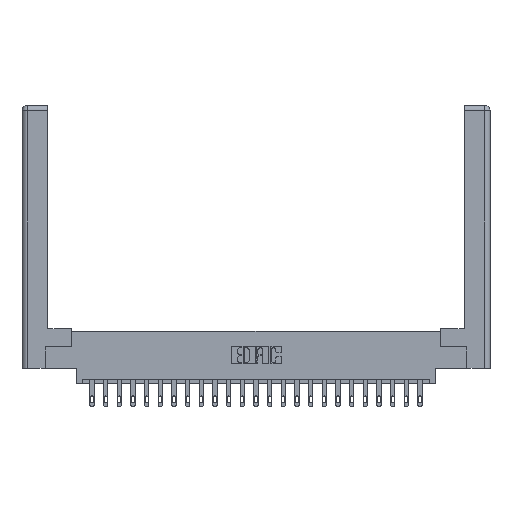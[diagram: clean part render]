
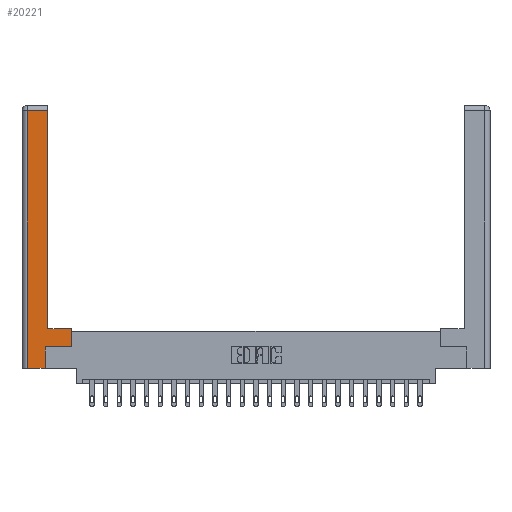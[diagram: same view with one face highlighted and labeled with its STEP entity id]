
A CAD part, top view. The second image highlights one B-rep face of the part: STEP entity #20221.
In plain terms, the highlighted planar face has unit normal (0, 0, 1).
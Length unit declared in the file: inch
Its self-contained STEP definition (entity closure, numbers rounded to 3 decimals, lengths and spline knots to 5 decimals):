
#418 = VECTOR ( 'NONE', #13907, 39.37008 ) ;
#998 = DIRECTION ( 'NONE',  ( 0., 0., -1. ) ) ;
#1299 = VECTOR ( 'NONE', #5932, 39.37008 ) ;
#1701 = LINE ( 'NONE', #20860, #18689 ) ;
#2306 = DIRECTION ( 'NONE',  ( 1., 0., 0. ) ) ;
#2366 = ORIENTED_EDGE ( 'NONE', *, *, #10690, .T. ) ;
#2379 = CARTESIAN_POINT ( 'NONE',  ( 0.565, 0.245, 0. ) ) ;
#2424 = VERTEX_POINT ( 'NONE', #11242 ) ;
#2531 = VERTEX_POINT ( 'NONE', #2379 ) ;
#2555 = EDGE_CURVE ( 'NONE', #7389, #2424, #16528, .T. ) ;
#3849 = DIRECTION ( 'NONE',  ( 0., 1., 0. ) ) ;
#3853 = FACE_OUTER_BOUND ( 'NONE', #3974, .T. ) ;
#3923 = CARTESIAN_POINT ( 'NONE',  ( 0.265, 0.245, 0. ) ) ;
#3974 = EDGE_LOOP ( 'NONE', ( #2366, #7760, #23906, #14959, #4752, #15238, #15988, #21761 ) ) ;
#4014 = CARTESIAN_POINT ( 'NONE',  ( 0.0615, 0., 0. ) ) ;
#4451 = CARTESIAN_POINT ( 'NONE',  ( 0.0615, 2.94, 0. ) ) ;
#4752 = ORIENTED_EDGE ( 'NONE', *, *, #21099, .T. ) ;
#5084 = EDGE_CURVE ( 'NONE', #19038, #7389, #6568, .T. ) ;
#5932 = DIRECTION ( 'NONE',  ( 0., 1., 0. ) ) ;
#6568 = LINE ( 'NONE', #4451, #418 ) ;
#7389 = VERTEX_POINT ( 'NONE', #16466 ) ;
#7545 = DIRECTION ( 'NONE',  ( 0., 1., 0. ) ) ;
#7642 = CARTESIAN_POINT ( 'NONE',  ( 0.265, 0., 0. ) ) ;
#7760 = ORIENTED_EDGE ( 'NONE', *, *, #5084, .T. ) ;
#8191 = VERTEX_POINT ( 'NONE', #22453 ) ;
#8256 = EDGE_CURVE ( 'NONE', #23671, #8191, #20503, .T. ) ;
#8374 = PLANE ( 'NONE',  #10267 ) ;
#8852 = CARTESIAN_POINT ( 'NONE',  ( 0.265, 0.245, 0. ) ) ;
#9056 = LINE ( 'NONE', #3923, #13434 ) ;
#9840 = DIRECTION ( 'NONE',  ( -1., 0., 0. ) ) ;
#10085 = VECTOR ( 'NONE', #2306, 39.37008 ) ;
#10267 = AXIS2_PLACEMENT_3D ( 'NONE', #16216, #998, #14243 ) ;
#10690 = EDGE_CURVE ( 'NONE', #8191, #19038, #10992, .T. ) ;
#10992 = LINE ( 'NONE', #15059, #1299 ) ;
#11045 = CARTESIAN_POINT ( 'NONE',  ( 0.295, 2.94, 0. ) ) ;
#11242 = CARTESIAN_POINT ( 'NONE',  ( 0.0615, 0., 0. ) ) ;
#13253 = CARTESIAN_POINT ( 'NONE',  ( 0.565, 0.45, 0. ) ) ;
#13434 = VECTOR ( 'NONE', #3849, 39.37008 ) ;
#13907 = DIRECTION ( 'NONE',  ( -1., 0., 0. ) ) ;
#14243 = DIRECTION ( 'NONE',  ( -1., 0., 0. ) ) ;
#14959 = ORIENTED_EDGE ( 'NONE', *, *, #18360, .T. ) ;
#15059 = CARTESIAN_POINT ( 'NONE',  ( 0.295, 3., 0. ) ) ;
#15110 = DIRECTION ( 'NONE',  ( 1., 0., 0. ) ) ;
#15238 = ORIENTED_EDGE ( 'NONE', *, *, #21223, .T. ) ;
#15934 = VERTEX_POINT ( 'NONE', #16147 ) ;
#15988 = ORIENTED_EDGE ( 'NONE', *, *, #16335, .T. ) ;
#16147 = CARTESIAN_POINT ( 'NONE',  ( 0.265, 0., 0. ) ) ;
#16216 = CARTESIAN_POINT ( 'NONE',  ( 0., 0., 0. ) ) ;
#16335 = EDGE_CURVE ( 'NONE', #2531, #23671, #18277, .T. ) ;
#16466 = CARTESIAN_POINT ( 'NONE',  ( 0.0615, 2.94, 0. ) ) ;
#16528 = LINE ( 'NONE', #4014, #23610 ) ;
#16723 = VERTEX_POINT ( 'NONE', #8852 ) ;
#17961 = LINE ( 'NONE', #7642, #10085 ) ;
#18277 = LINE ( 'NONE', #22723, #20930 ) ;
#18360 = EDGE_CURVE ( 'NONE', #2424, #15934, #17961, .T. ) ;
#18689 = VECTOR ( 'NONE', #15110, 39.37008 ) ;
#19038 = VERTEX_POINT ( 'NONE', #11045 ) ;
#19335 = VECTOR ( 'NONE', #9840, 39.37008 ) ;
#20221 = ADVANCED_FACE ( 'NONE', ( #3853 ), #8374, .F. ) ;
#20503 = LINE ( 'NONE', #21038, #19335 ) ;
#20860 = CARTESIAN_POINT ( 'NONE',  ( 0.565, 0.245, 0. ) ) ;
#20930 = VECTOR ( 'NONE', #7545, 39.37008 ) ;
#20956 = DIRECTION ( 'NONE',  ( 0., -1., 0. ) ) ;
#21038 = CARTESIAN_POINT ( 'NONE',  ( 0.295, 0.45, 0. ) ) ;
#21099 = EDGE_CURVE ( 'NONE', #15934, #16723, #9056, .T. ) ;
#21223 = EDGE_CURVE ( 'NONE', #16723, #2531, #1701, .T. ) ;
#21761 = ORIENTED_EDGE ( 'NONE', *, *, #8256, .T. ) ;
#22453 = CARTESIAN_POINT ( 'NONE',  ( 0.295, 0.45, 0. ) ) ;
#22723 = CARTESIAN_POINT ( 'NONE',  ( 0.565, 0.45, 0. ) ) ;
#23610 = VECTOR ( 'NONE', #20956, 39.37008 ) ;
#23671 = VERTEX_POINT ( 'NONE', #13253 ) ;
#23906 = ORIENTED_EDGE ( 'NONE', *, *, #2555, .T. ) ;
